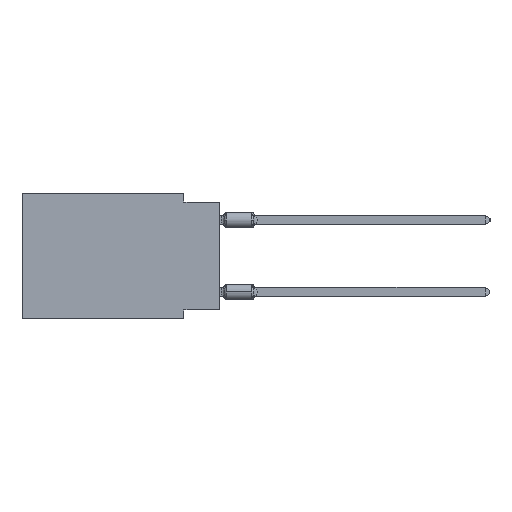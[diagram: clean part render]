
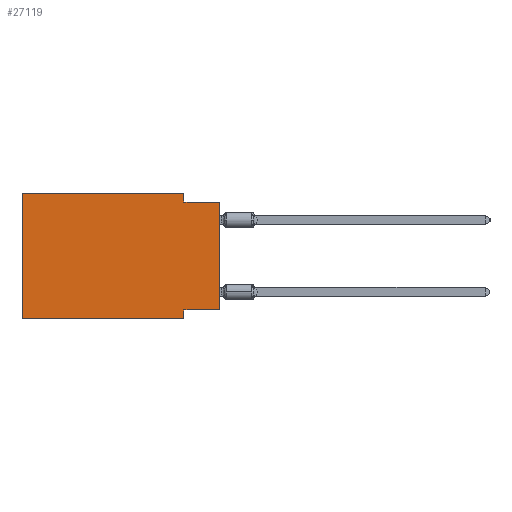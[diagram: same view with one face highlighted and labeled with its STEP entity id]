
A CAD part, left-side view. The second image highlights one B-rep face of the part: STEP entity #27119.
In plain terms, the highlighted planar face has unit normal (-1, 0, 0).
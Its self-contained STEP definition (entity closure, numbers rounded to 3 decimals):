
#644 = CARTESIAN_POINT ( 'NONE',  ( 0., 2.54, -0.635 ) ) ;
#658 = EDGE_CURVE ( 'NONE', #49559, #31152, #12767, .T. ) ;
#2163 = CARTESIAN_POINT ( 'NONE',  ( 0., 2.54, -8.255 ) ) ;
#2434 = PLANE ( 'NONE',  #14474 ) ;
#2717 = CARTESIAN_POINT ( 'NONE',  ( 0., 0., -0.635 ) ) ;
#2840 = LINE ( 'NONE', #3700, #35107 ) ;
#3700 = CARTESIAN_POINT ( 'NONE',  ( 0., 13.97, 0. ) ) ;
#3929 = DIRECTION ( 'NONE',  ( 0., 0., -1. ) ) ;
#4118 = ORIENTED_EDGE ( 'NONE', *, *, #35148, .F. ) ;
#4225 = LINE ( 'NONE', #26348, #22517 ) ;
#4742 = CARTESIAN_POINT ( 'NONE',  ( 0., 2.54, 0. ) ) ;
#5965 = CARTESIAN_POINT ( 'NONE',  ( 0., 13.97, 0. ) ) ;
#6965 = CARTESIAN_POINT ( 'NONE',  ( 0., 0., -0.635 ) ) ;
#8596 = CARTESIAN_POINT ( 'NONE',  ( 0., 13.97, 0. ) ) ;
#10625 = VERTEX_POINT ( 'NONE', #5965 ) ;
#11346 = CARTESIAN_POINT ( 'NONE',  ( 0., 13.97, -8.89 ) ) ;
#12767 = LINE ( 'NONE', #43445, #46455 ) ;
#13200 = EDGE_CURVE ( 'NONE', #44395, #13975, #48016, .T. ) ;
#13975 = VERTEX_POINT ( 'NONE', #2163 ) ;
#14474 = AXIS2_PLACEMENT_3D ( 'NONE', #8596, #18320, #17755 ) ;
#17089 = CARTESIAN_POINT ( 'NONE',  ( 0., 2.54, -8.89 ) ) ;
#17571 = CARTESIAN_POINT ( 'NONE',  ( 0., 2.54, 0. ) ) ;
#17755 = DIRECTION ( 'NONE',  ( 0., 0., -1. ) ) ;
#18320 = DIRECTION ( 'NONE',  ( 1., 0., 0. ) ) ;
#18898 = VECTOR ( 'NONE', #21478, 1000. ) ;
#21187 = CARTESIAN_POINT ( 'NONE',  ( 0., 0., -8.255 ) ) ;
#21478 = DIRECTION ( 'NONE',  ( 0., 1., 0. ) ) ;
#22459 = DIRECTION ( 'NONE',  ( 0., 0., -1. ) ) ;
#22517 = VECTOR ( 'NONE', #3929, 1000. ) ;
#23049 = ORIENTED_EDGE ( 'NONE', *, *, #35371, .F. ) ;
#24841 = DIRECTION ( 'NONE',  ( 0., -1., 0. ) ) ;
#25452 = ORIENTED_EDGE ( 'NONE', *, *, #13200, .F. ) ;
#25740 = DIRECTION ( 'NONE',  ( 0., -1., 0. ) ) ;
#26348 = CARTESIAN_POINT ( 'NONE',  ( 0., 2.54, -8.89 ) ) ;
#26771 = EDGE_CURVE ( 'NONE', #33551, #34125, #48998, .T. ) ;
#27119 = ADVANCED_FACE ( 'NONE', ( #42843 ), #2434, .F. ) ;
#27225 = VECTOR ( 'NONE', #24841, 1000. ) ;
#27927 = CARTESIAN_POINT ( 'NONE',  ( 0., 13.97, 0. ) ) ;
#30582 = EDGE_CURVE ( 'NONE', #44395, #56547, #38485, .T. ) ;
#31152 = VERTEX_POINT ( 'NONE', #17089 ) ;
#31895 = CARTESIAN_POINT ( 'NONE',  ( 0., 0., -8.255 ) ) ;
#33112 = LINE ( 'NONE', #2717, #27225 ) ;
#33551 = VERTEX_POINT ( 'NONE', #17571 ) ;
#34125 = VERTEX_POINT ( 'NONE', #644 ) ;
#35107 = VECTOR ( 'NONE', #48244, 1000. ) ;
#35143 = VECTOR ( 'NONE', #22459, 1000. ) ;
#35148 = EDGE_CURVE ( 'NONE', #13975, #31152, #4225, .T. ) ;
#35371 = EDGE_CURVE ( 'NONE', #34125, #56547, #33112, .T. ) ;
#36787 = ORIENTED_EDGE ( 'NONE', *, *, #30582, .T. ) ;
#38485 = LINE ( 'NONE', #42335, #50538 ) ;
#40016 = ORIENTED_EDGE ( 'NONE', *, *, #49175, .F. ) ;
#42335 = CARTESIAN_POINT ( 'NONE',  ( 0., 0., 0. ) ) ;
#42843 = FACE_OUTER_BOUND ( 'NONE', #47388, .T. ) ;
#43445 = CARTESIAN_POINT ( 'NONE',  ( 0., 13.97, -8.89 ) ) ;
#44395 = VERTEX_POINT ( 'NONE', #31895 ) ;
#45326 = LINE ( 'NONE', #27927, #50522 ) ;
#45627 = DIRECTION ( 'NONE',  ( 0., 0., 1. ) ) ;
#46455 = VECTOR ( 'NONE', #25740, 1000. ) ;
#47388 = EDGE_LOOP ( 'NONE', ( #36787, #23049, #51766, #40016, #48841, #52084, #4118, #25452 ) ) ;
#48016 = LINE ( 'NONE', #21187, #18898 ) ;
#48244 = DIRECTION ( 'NONE',  ( 0., -1., 0. ) ) ;
#48841 = ORIENTED_EDGE ( 'NONE', *, *, #57725, .F. ) ;
#48998 = LINE ( 'NONE', #4742, #35143 ) ;
#49175 = EDGE_CURVE ( 'NONE', #10625, #33551, #2840, .T. ) ;
#49559 = VERTEX_POINT ( 'NONE', #11346 ) ;
#50522 = VECTOR ( 'NONE', #45627, 1000. ) ;
#50538 = VECTOR ( 'NONE', #55891, 1000. ) ;
#51766 = ORIENTED_EDGE ( 'NONE', *, *, #26771, .F. ) ;
#52084 = ORIENTED_EDGE ( 'NONE', *, *, #658, .T. ) ;
#55891 = DIRECTION ( 'NONE',  ( 0., 0., 1. ) ) ;
#56547 = VERTEX_POINT ( 'NONE', #6965 ) ;
#57725 = EDGE_CURVE ( 'NONE', #49559, #10625, #45326, .T. ) ;
